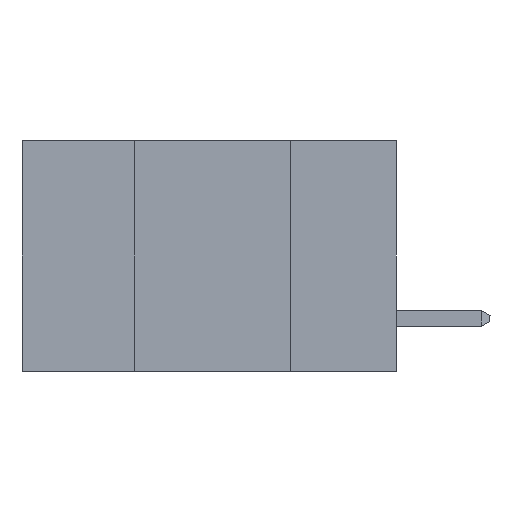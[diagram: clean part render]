
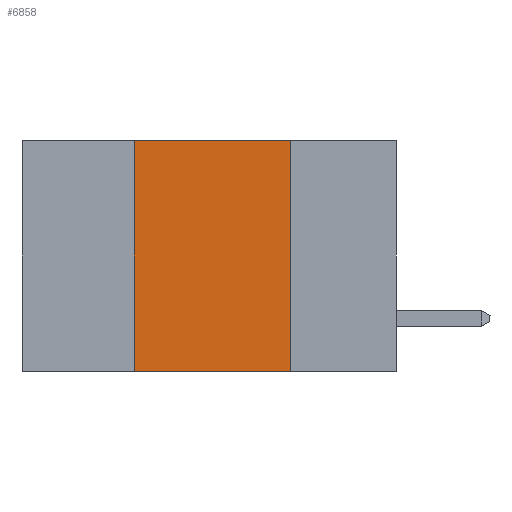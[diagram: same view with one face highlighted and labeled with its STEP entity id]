
A CAD part, left-side view. The second image highlights one B-rep face of the part: STEP entity #6858.
In plain terms, the highlighted planar face has unit normal (-1, 0, 0).
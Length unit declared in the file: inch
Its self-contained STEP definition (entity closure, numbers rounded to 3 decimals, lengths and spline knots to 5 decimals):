
#403 = CARTESIAN_POINT ( 'NONE',  ( 0., 0.6, 0. ) ) ;
#423 = LINE ( 'NONE', #5026, #5834 ) ;
#585 = CARTESIAN_POINT ( 'NONE',  ( 0., 0.6, -0.37 ) ) ;
#816 = EDGE_CURVE ( 'NONE', #5157, #2595, #7126, .T. ) ;
#903 = LINE ( 'NONE', #585, #8054 ) ;
#949 = VERTEX_POINT ( 'NONE', #8130 ) ;
#1174 = ORIENTED_EDGE ( 'NONE', *, *, #1418, .F. ) ;
#1245 = AXIS2_PLACEMENT_3D ( 'NONE', #2921, #3629, #8389 ) ;
#1418 = EDGE_CURVE ( 'NONE', #2595, #3171, #423, .T. ) ;
#2181 = CARTESIAN_POINT ( 'NONE',  ( 0., 0.17, -0.37 ) ) ;
#2267 = EDGE_LOOP ( 'NONE', ( #1174, #6977, #6446, #3202 ) ) ;
#2595 = VERTEX_POINT ( 'NONE', #8505 ) ;
#2921 = CARTESIAN_POINT ( 'NONE',  ( 0., 0.6, 0. ) ) ;
#3171 = VERTEX_POINT ( 'NONE', #2181 ) ;
#3202 = ORIENTED_EDGE ( 'NONE', *, *, #7336, .T. ) ;
#3374 = VECTOR ( 'NONE', #5450, 39.37008 ) ;
#3629 = DIRECTION ( 'NONE',  ( 1., 0., 0. ) ) ;
#3700 = VECTOR ( 'NONE', #4686, 39.37008 ) ;
#3756 = CARTESIAN_POINT ( 'NONE',  ( 0., 0.42, 0. ) ) ;
#4115 = DIRECTION ( 'NONE',  ( 0., -1., 0. ) ) ;
#4686 = DIRECTION ( 'NONE',  ( 0., -1., 0. ) ) ;
#5026 = CARTESIAN_POINT ( 'NONE',  ( 0., 0.17, -0.37 ) ) ;
#5035 = LINE ( 'NONE', #5457, #3374 ) ;
#5157 = VERTEX_POINT ( 'NONE', #3756 ) ;
#5286 = DIRECTION ( 'NONE',  ( 0., 0., -1. ) ) ;
#5450 = DIRECTION ( 'NONE',  ( 0., 0., 1. ) ) ;
#5457 = CARTESIAN_POINT ( 'NONE',  ( 0., 0.42, -0.37 ) ) ;
#5834 = VECTOR ( 'NONE', #5286, 39.37008 ) ;
#5931 = EDGE_CURVE ( 'NONE', #949, #5157, #5035, .T. ) ;
#6446 = ORIENTED_EDGE ( 'NONE', *, *, #5931, .F. ) ;
#6858 = ADVANCED_FACE ( 'NONE', ( #6930 ), #7713, .F. ) ;
#6930 = FACE_OUTER_BOUND ( 'NONE', #2267, .T. ) ;
#6977 = ORIENTED_EDGE ( 'NONE', *, *, #816, .F. ) ;
#7126 = LINE ( 'NONE', #403, #3700 ) ;
#7336 = EDGE_CURVE ( 'NONE', #949, #3171, #903, .T. ) ;
#7713 = PLANE ( 'NONE',  #1245 ) ;
#8054 = VECTOR ( 'NONE', #4115, 39.37008 ) ;
#8130 = CARTESIAN_POINT ( 'NONE',  ( 0., 0.42, -0.37 ) ) ;
#8389 = DIRECTION ( 'NONE',  ( 0., 0., -1. ) ) ;
#8505 = CARTESIAN_POINT ( 'NONE',  ( 0., 0.17, 0. ) ) ;
